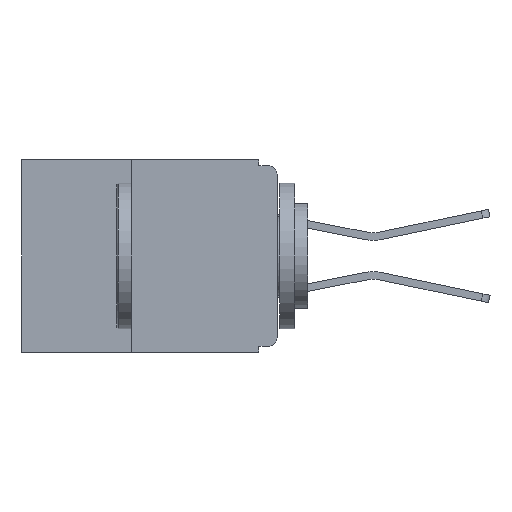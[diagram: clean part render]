
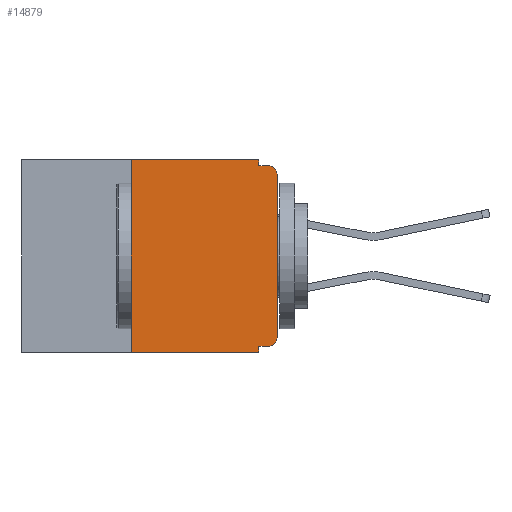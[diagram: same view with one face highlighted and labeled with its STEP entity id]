
A CAD part, left-side view. The second image highlights one B-rep face of the part: STEP entity #14879.
In plain terms, the highlighted planar face has unit normal (-1, 0, 0).
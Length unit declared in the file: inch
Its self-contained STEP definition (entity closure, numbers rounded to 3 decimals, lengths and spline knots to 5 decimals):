
#113 = EDGE_CURVE ( 'NONE', #1197, #15924, #11825, .T. ) ;
#172 = CARTESIAN_POINT ( 'NONE',  ( 0., 0.25, 0. ) ) ;
#446 = VERTEX_POINT ( 'NONE', #14455 ) ;
#865 = DIRECTION ( 'NONE',  ( 0., 0., -1. ) ) ;
#1052 = CARTESIAN_POINT ( 'NONE',  ( 0., 0.015, -0.01 ) ) ;
#1197 = VERTEX_POINT ( 'NONE', #5490 ) ;
#1225 = ORIENTED_EDGE ( 'NONE', *, *, #17907, .F. ) ;
#1383 = CARTESIAN_POINT ( 'NONE',  ( 0., 0.031, 0. ) ) ;
#1595 = EDGE_CURVE ( 'NONE', #17829, #446, #2627, .T. ) ;
#2102 = CIRCLE ( 'NONE', #2282, 0.015 ) ;
#2199 = EDGE_CURVE ( 'NONE', #446, #16232, #16293, .T. ) ;
#2282 = AXIS2_PLACEMENT_3D ( 'NONE', #18113, #18082, #18055 ) ;
#2353 = VERTEX_POINT ( 'NONE', #172 ) ;
#2411 = CARTESIAN_POINT ( 'NONE',  ( 0., 0., -0.01 ) ) ;
#2627 = CIRCLE ( 'NONE', #16980, 0.015 ) ;
#3484 = LINE ( 'NONE', #10021, #14659 ) ;
#3990 = EDGE_CURVE ( 'NONE', #1197, #2353, #15603, .T. ) ;
#4566 = DIRECTION ( 'NONE',  ( 0., 0., -1. ) ) ;
#4891 = EDGE_CURVE ( 'NONE', #2353, #5268, #12193, .T. ) ;
#4940 = EDGE_CURVE ( 'NONE', #5268, #6419, #3484, .T. ) ;
#5046 = VERTEX_POINT ( 'NONE', #7206 ) ;
#5085 = DIRECTION ( 'NONE',  ( 0., -1., 0. ) ) ;
#5268 = VERTEX_POINT ( 'NONE', #1383 ) ;
#5428 = EDGE_CURVE ( 'NONE', #16232, #14978, #2102, .T. ) ;
#5490 = CARTESIAN_POINT ( 'NONE',  ( 0., 0.25, -0.33 ) ) ;
#6181 = ORIENTED_EDGE ( 'NONE', *, *, #2199, .T. ) ;
#6353 = VECTOR ( 'NONE', #14079, 39.37008 ) ;
#6419 = VERTEX_POINT ( 'NONE', #9738 ) ;
#7206 = CARTESIAN_POINT ( 'NONE',  ( 0., 0.031, -0.32 ) ) ;
#8094 = VECTOR ( 'NONE', #8539, 39.37008 ) ;
#8209 = AXIS2_PLACEMENT_3D ( 'NONE', #16764, #9545, #865 ) ;
#8348 = CARTESIAN_POINT ( 'NONE',  ( 0., 0., -0.025 ) ) ;
#8384 = EDGE_CURVE ( 'NONE', #17829, #5046, #9296, .T. ) ;
#8539 = DIRECTION ( 'NONE',  ( 0., 0., 1. ) ) ;
#9038 = DIRECTION ( 'NONE',  ( 0., 0., -1. ) ) ;
#9093 = DIRECTION ( 'NONE',  ( -1., 0., 0. ) ) ;
#9296 = LINE ( 'NONE', #17957, #10243 ) ;
#9545 = DIRECTION ( 'NONE',  ( 1., 0., 0. ) ) ;
#9738 = CARTESIAN_POINT ( 'NONE',  ( 0., 0.031, -0.01 ) ) ;
#10021 = CARTESIAN_POINT ( 'NONE',  ( 0., 0.031, 0. ) ) ;
#10092 = DIRECTION ( 'NONE',  ( 0., 0., -1. ) ) ;
#10243 = VECTOR ( 'NONE', #18017, 39.37008 ) ;
#11032 = ORIENTED_EDGE ( 'NONE', *, *, #14284, .F. ) ;
#11369 = FACE_OUTER_BOUND ( 'NONE', #16937, .T. ) ;
#11485 = CARTESIAN_POINT ( 'NONE',  ( 0., 0.437, 0. ) ) ;
#11492 = ORIENTED_EDGE ( 'NONE', *, *, #4891, .F. ) ;
#11493 = CARTESIAN_POINT ( 'NONE',  ( 0., 0.015, -0.305 ) ) ;
#11677 = DIRECTION ( 'NONE',  ( 0., -1., 0. ) ) ;
#11699 = CARTESIAN_POINT ( 'NONE',  ( 0., 0.015, -0.32 ) ) ;
#11825 = LINE ( 'NONE', #17833, #15212 ) ;
#11990 = DIRECTION ( 'NONE',  ( 0., 0., 1. ) ) ;
#12048 = CARTESIAN_POINT ( 'NONE',  ( 0., 0.25, -0.33 ) ) ;
#12162 = CARTESIAN_POINT ( 'NONE',  ( 0., 0., 0. ) ) ;
#12193 = LINE ( 'NONE', #11485, #15564 ) ;
#12232 = VECTOR ( 'NONE', #11990, 39.37008 ) ;
#12398 = ORIENTED_EDGE ( 'NONE', *, *, #113, .T. ) ;
#12843 = ORIENTED_EDGE ( 'NONE', *, *, #8384, .F. ) ;
#14079 = DIRECTION ( 'NONE',  ( 0., -1., 0. ) ) ;
#14284 = EDGE_CURVE ( 'NONE', #6419, #14978, #14604, .T. ) ;
#14455 = CARTESIAN_POINT ( 'NONE',  ( 0., 0., -0.305 ) ) ;
#14604 = LINE ( 'NONE', #2411, #6353 ) ;
#14659 = VECTOR ( 'NONE', #10092, 39.37008 ) ;
#14784 = CARTESIAN_POINT ( 'NONE',  ( 0., 0.031, -0.33 ) ) ;
#14879 = ADVANCED_FACE ( 'NONE', ( #11369 ), #15363, .F. ) ;
#14888 = ORIENTED_EDGE ( 'NONE', *, *, #4940, .F. ) ;
#14898 = CARTESIAN_POINT ( 'NONE',  ( 0., 0.031, -0.33 ) ) ;
#14905 = VECTOR ( 'NONE', #4566, 39.37008 ) ;
#14978 = VERTEX_POINT ( 'NONE', #1052 ) ;
#15212 = VECTOR ( 'NONE', #5085, 39.37008 ) ;
#15328 = ORIENTED_EDGE ( 'NONE', *, *, #3990, .F. ) ;
#15342 = LINE ( 'NONE', #14784, #14905 ) ;
#15363 = PLANE ( 'NONE',  #8209 ) ;
#15564 = VECTOR ( 'NONE', #11677, 39.37008 ) ;
#15603 = LINE ( 'NONE', #12048, #12232 ) ;
#15924 = VERTEX_POINT ( 'NONE', #14898 ) ;
#16232 = VERTEX_POINT ( 'NONE', #8348 ) ;
#16293 = LINE ( 'NONE', #12162, #8094 ) ;
#16638 = ORIENTED_EDGE ( 'NONE', *, *, #1595, .T. ) ;
#16764 = CARTESIAN_POINT ( 'NONE',  ( 0., 0.437, 0. ) ) ;
#16937 = EDGE_LOOP ( 'NONE', ( #6181, #18125, #11032, #14888, #11492, #15328, #12398, #1225, #12843, #16638 ) ) ;
#16980 = AXIS2_PLACEMENT_3D ( 'NONE', #11493, #9093, #9038 ) ;
#17829 = VERTEX_POINT ( 'NONE', #11699 ) ;
#17833 = CARTESIAN_POINT ( 'NONE',  ( 0., 0.437, -0.33 ) ) ;
#17907 = EDGE_CURVE ( 'NONE', #5046, #15924, #15342, .T. ) ;
#17957 = CARTESIAN_POINT ( 'NONE',  ( 0., 0., -0.32 ) ) ;
#18017 = DIRECTION ( 'NONE',  ( 0., 1., 0. ) ) ;
#18055 = DIRECTION ( 'NONE',  ( 0., 0., -1. ) ) ;
#18082 = DIRECTION ( 'NONE',  ( -1., 0., 0. ) ) ;
#18113 = CARTESIAN_POINT ( 'NONE',  ( 0., 0.015, -0.025 ) ) ;
#18125 = ORIENTED_EDGE ( 'NONE', *, *, #5428, .T. ) ;
